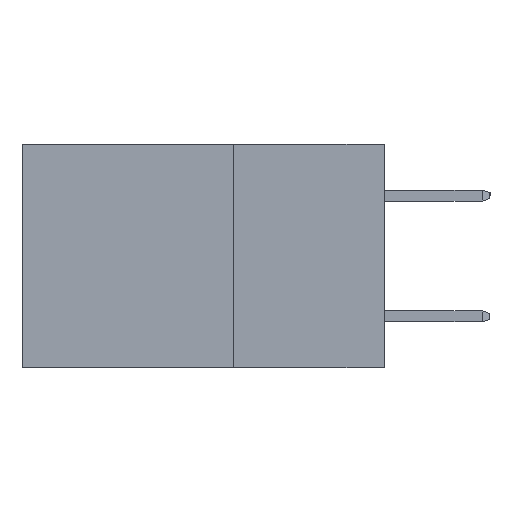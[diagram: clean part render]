
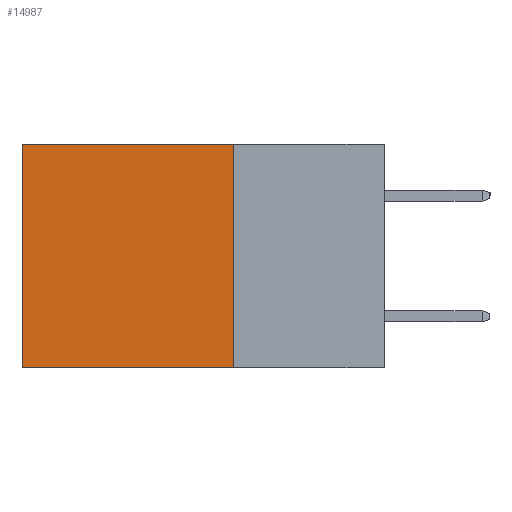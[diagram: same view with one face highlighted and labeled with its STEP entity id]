
A CAD part, left-side view. The second image highlights one B-rep face of the part: STEP entity #14987.
In plain terms, the highlighted planar face has unit normal (-1, 0, 0).
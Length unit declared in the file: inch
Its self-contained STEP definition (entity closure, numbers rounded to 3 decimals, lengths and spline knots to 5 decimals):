
#1687 = EDGE_CURVE ( 'NONE', #18972, #15152, #17443, .T. ) ;
#2074 = CARTESIAN_POINT ( 'NONE',  ( 0.2615, 0.6, -0.37 ) ) ;
#2651 = LINE ( 'NONE', #5767, #12747 ) ;
#2699 = VERTEX_POINT ( 'NONE', #3961 ) ;
#3215 = CARTESIAN_POINT ( 'NONE',  ( 0.2615, 0.25, 0. ) ) ;
#3961 = CARTESIAN_POINT ( 'NONE',  ( 0.2615, 0.25, -0.37 ) ) ;
#4431 = VERTEX_POINT ( 'NONE', #2074 ) ;
#4620 = ORIENTED_EDGE ( 'NONE', *, *, #14882, .F. ) ;
#5767 = CARTESIAN_POINT ( 'NONE',  ( 0.2615, 0.25, -0.37 ) ) ;
#5966 = CARTESIAN_POINT ( 'NONE',  ( 0.2615, 0.25, -0.37 ) ) ;
#7917 = DIRECTION ( 'NONE',  ( 1., 0., 0. ) ) ;
#8750 = ORIENTED_EDGE ( 'NONE', *, *, #20054, .F. ) ;
#9000 = VECTOR ( 'NONE', #9549, 39.37008 ) ;
#9549 = DIRECTION ( 'NONE',  ( 0., 1., 0. ) ) ;
#9592 = EDGE_LOOP ( 'NONE', ( #13466, #8750, #4620, #16065 ) ) ;
#10604 = DIRECTION ( 'NONE',  ( 0., 1., 0. ) ) ;
#11006 = CARTESIAN_POINT ( 'NONE',  ( 0.2615, 0.25, 0. ) ) ;
#11526 = LINE ( 'NONE', #13715, #18197 ) ;
#12102 = CARTESIAN_POINT ( 'NONE',  ( 0.2615, 0.6, -0.37 ) ) ;
#12747 = VECTOR ( 'NONE', #20243, 39.37008 ) ;
#13466 = ORIENTED_EDGE ( 'NONE', *, *, #14856, .T. ) ;
#13545 = PLANE ( 'NONE',  #17743 ) ;
#13715 = CARTESIAN_POINT ( 'NONE',  ( 0.2615, 0.25, -0.37 ) ) ;
#13857 = FACE_OUTER_BOUND ( 'NONE', #9592, .T. ) ;
#14163 = DIRECTION ( 'NONE',  ( 0., 0., -1. ) ) ;
#14764 = CARTESIAN_POINT ( 'NONE',  ( 0.2615, 0.6, 0. ) ) ;
#14856 = EDGE_CURVE ( 'NONE', #15152, #4431, #16672, .T. ) ;
#14882 = EDGE_CURVE ( 'NONE', #18972, #2699, #2651, .T. ) ;
#14987 = ADVANCED_FACE ( 'NONE', ( #13857 ), #13545, .F. ) ;
#15152 = VERTEX_POINT ( 'NONE', #14764 ) ;
#15512 = DIRECTION ( 'NONE',  ( 0., 0., -1. ) ) ;
#16065 = ORIENTED_EDGE ( 'NONE', *, *, #1687, .T. ) ;
#16672 = LINE ( 'NONE', #12102, #19043 ) ;
#17443 = LINE ( 'NONE', #3215, #9000 ) ;
#17743 = AXIS2_PLACEMENT_3D ( 'NONE', #5966, #7917, #14163 ) ;
#18197 = VECTOR ( 'NONE', #10604, 39.37008 ) ;
#18972 = VERTEX_POINT ( 'NONE', #11006 ) ;
#19043 = VECTOR ( 'NONE', #15512, 39.37008 ) ;
#20054 = EDGE_CURVE ( 'NONE', #2699, #4431, #11526, .T. ) ;
#20243 = DIRECTION ( 'NONE',  ( 0., 0., -1. ) ) ;
